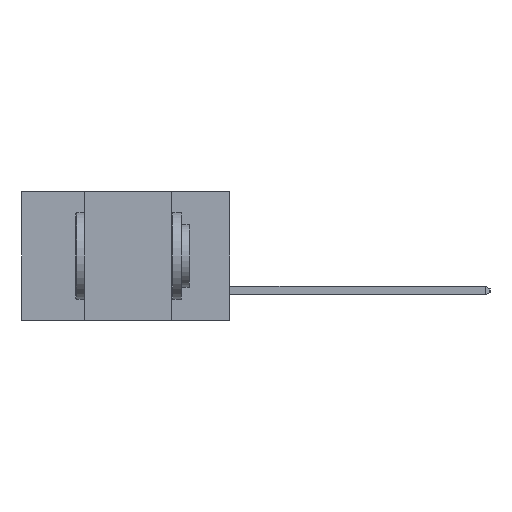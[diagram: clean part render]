
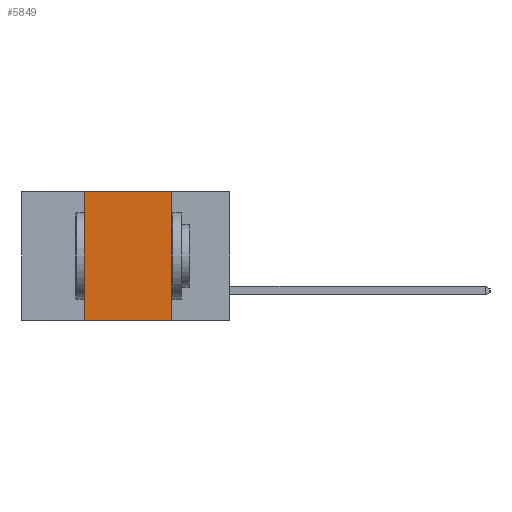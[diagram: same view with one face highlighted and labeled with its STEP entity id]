
A CAD part, left-side view. The second image highlights one B-rep face of the part: STEP entity #5849.
In plain terms, the highlighted planar face has unit normal (-1, 0, 0).
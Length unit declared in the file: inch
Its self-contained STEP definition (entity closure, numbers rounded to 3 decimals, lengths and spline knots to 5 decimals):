
#431 = VERTEX_POINT ( 'NONE', #17904 ) ;
#553 = LINE ( 'NONE', #15060, #14916 ) ;
#3584 = VECTOR ( 'NONE', #14941, 39.37008 ) ;
#4856 = CARTESIAN_POINT ( 'NONE',  ( 0., 0.42, 0. ) ) ;
#5849 = ADVANCED_FACE ( 'NONE', ( #6013 ), #20370, .F. ) ;
#5886 = EDGE_CURVE ( 'NONE', #13523, #431, #553, .T. ) ;
#6013 = FACE_OUTER_BOUND ( 'NONE', #16647, .T. ) ;
#6044 = ORIENTED_EDGE ( 'NONE', *, *, #10653, .F. ) ;
#6340 = VECTOR ( 'NONE', #16161, 39.37008 ) ;
#8254 = EDGE_CURVE ( 'NONE', #13523, #19841, #19206, .T. ) ;
#8904 = LINE ( 'NONE', #15058, #3584 ) ;
#9449 = EDGE_CURVE ( 'NONE', #19841, #15515, #8904, .T. ) ;
#10653 = EDGE_CURVE ( 'NONE', #15515, #431, #19350, .T. ) ;
#11631 = AXIS2_PLACEMENT_3D ( 'NONE', #20484, #20351, #17992 ) ;
#12461 = ORIENTED_EDGE ( 'NONE', *, *, #5886, .T. ) ;
#13523 = VERTEX_POINT ( 'NONE', #21162 ) ;
#14531 = VECTOR ( 'NONE', #18719, 39.37008 ) ;
#14916 = VECTOR ( 'NONE', #15251, 39.37008 ) ;
#14941 = DIRECTION ( 'NONE',  ( 0., -1., 0. ) ) ;
#15058 = CARTESIAN_POINT ( 'NONE',  ( 0., 0.6, 0. ) ) ;
#15060 = CARTESIAN_POINT ( 'NONE',  ( 0., 0.6, -0.37 ) ) ;
#15251 = DIRECTION ( 'NONE',  ( 0., -1., 0. ) ) ;
#15515 = VERTEX_POINT ( 'NONE', #20052 ) ;
#16127 = CARTESIAN_POINT ( 'NONE',  ( 0., 0.17, -0.37 ) ) ;
#16161 = DIRECTION ( 'NONE',  ( 0., 0., -1. ) ) ;
#16617 = ORIENTED_EDGE ( 'NONE', *, *, #8254, .F. ) ;
#16647 = EDGE_LOOP ( 'NONE', ( #6044, #20125, #16617, #12461 ) ) ;
#17904 = CARTESIAN_POINT ( 'NONE',  ( 0., 0.17, -0.37 ) ) ;
#17919 = CARTESIAN_POINT ( 'NONE',  ( 0., 0.42, -0.37 ) ) ;
#17992 = DIRECTION ( 'NONE',  ( 0., 0., -1. ) ) ;
#18719 = DIRECTION ( 'NONE',  ( 0., 0., 1. ) ) ;
#19206 = LINE ( 'NONE', #17919, #14531 ) ;
#19350 = LINE ( 'NONE', #16127, #6340 ) ;
#19841 = VERTEX_POINT ( 'NONE', #4856 ) ;
#20052 = CARTESIAN_POINT ( 'NONE',  ( 0., 0.17, 0. ) ) ;
#20125 = ORIENTED_EDGE ( 'NONE', *, *, #9449, .F. ) ;
#20351 = DIRECTION ( 'NONE',  ( 1., 0., 0. ) ) ;
#20370 = PLANE ( 'NONE',  #11631 ) ;
#20484 = CARTESIAN_POINT ( 'NONE',  ( 0., 0.6, 0. ) ) ;
#21162 = CARTESIAN_POINT ( 'NONE',  ( 0., 0.42, -0.37 ) ) ;
